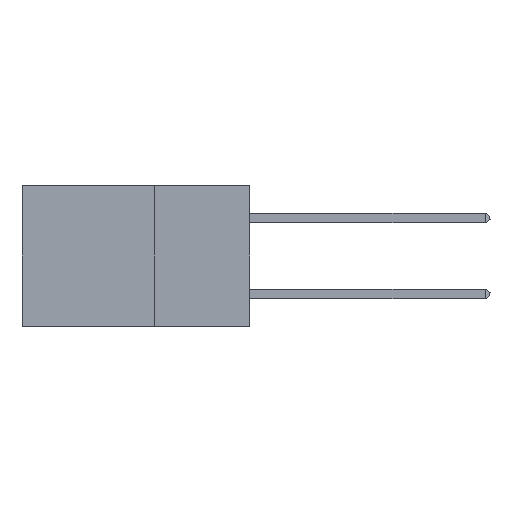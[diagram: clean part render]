
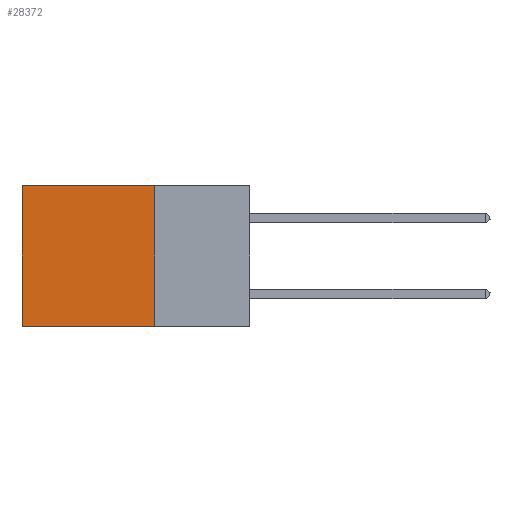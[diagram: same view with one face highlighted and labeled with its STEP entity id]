
A CAD part, left-side view. The second image highlights one B-rep face of the part: STEP entity #28372.
In plain terms, the highlighted planar face has unit normal (-1, 0, 0).
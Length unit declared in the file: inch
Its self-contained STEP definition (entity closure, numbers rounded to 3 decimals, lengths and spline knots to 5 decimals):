
#21 = VECTOR ( 'NONE', #28207, 39.37008 ) ;
#1309 = ORIENTED_EDGE ( 'NONE', *, *, #24073, .F. ) ;
#2085 = CARTESIAN_POINT ( 'NONE',  ( 0.2875, 0.25, -0.37 ) ) ;
#2307 = CARTESIAN_POINT ( 'NONE',  ( 0.2875, 0.6, -0.37 ) ) ;
#4442 = CARTESIAN_POINT ( 'NONE',  ( 0.2875, 0.6, 0. ) ) ;
#6244 = CARTESIAN_POINT ( 'NONE',  ( 0.2875, 0.6, 0. ) ) ;
#6310 = VECTOR ( 'NONE', #12137, 39.37008 ) ;
#8780 = EDGE_CURVE ( 'NONE', #23820, #26030, #32071, .T. ) ;
#9561 = FACE_OUTER_BOUND ( 'NONE', #30292, .T. ) ;
#12137 = DIRECTION ( 'NONE',  ( 0., 0., -1. ) ) ;
#13172 = CARTESIAN_POINT ( 'NONE',  ( 0.2875, 0.25, 0. ) ) ;
#13196 = VECTOR ( 'NONE', #37421, 39.37008 ) ;
#14768 = ORIENTED_EDGE ( 'NONE', *, *, #31474, .T. ) ;
#14882 = VERTEX_POINT ( 'NONE', #2085 ) ;
#15533 = DIRECTION ( 'NONE',  ( 0., 0., -1. ) ) ;
#16046 = ORIENTED_EDGE ( 'NONE', *, *, #35942, .F. ) ;
#16591 = CARTESIAN_POINT ( 'NONE',  ( 0.2875, 0.25, -0.37 ) ) ;
#17099 = ORIENTED_EDGE ( 'NONE', *, *, #8780, .T. ) ;
#18482 = CARTESIAN_POINT ( 'NONE',  ( 0.2875, 0.25, 0. ) ) ;
#20357 = LINE ( 'NONE', #16591, #13196 ) ;
#21575 = PLANE ( 'NONE',  #27815 ) ;
#22110 = LINE ( 'NONE', #6244, #30879 ) ;
#23820 = VERTEX_POINT ( 'NONE', #34903 ) ;
#24073 = EDGE_CURVE ( 'NONE', #23820, #14882, #38143, .T. ) ;
#26030 = VERTEX_POINT ( 'NONE', #4442 ) ;
#26228 = VERTEX_POINT ( 'NONE', #2307 ) ;
#27205 = CARTESIAN_POINT ( 'NONE',  ( 0.2875, 0.25, 0. ) ) ;
#27389 = DIRECTION ( 'NONE',  ( 0., 0., -1. ) ) ;
#27815 = AXIS2_PLACEMENT_3D ( 'NONE', #18482, #33432, #15533 ) ;
#28207 = DIRECTION ( 'NONE',  ( 0., 1., 0. ) ) ;
#28372 = ADVANCED_FACE ( 'NONE', ( #9561 ), #21575, .F. ) ;
#30292 = EDGE_LOOP ( 'NONE', ( #14768, #16046, #1309, #17099 ) ) ;
#30879 = VECTOR ( 'NONE', #27389, 39.37008 ) ;
#31474 = EDGE_CURVE ( 'NONE', #26030, #26228, #22110, .T. ) ;
#32071 = LINE ( 'NONE', #13172, #21 ) ;
#33432 = DIRECTION ( 'NONE',  ( 1., 0., 0. ) ) ;
#34903 = CARTESIAN_POINT ( 'NONE',  ( 0.2875, 0.25, 0. ) ) ;
#35942 = EDGE_CURVE ( 'NONE', #14882, #26228, #20357, .T. ) ;
#37421 = DIRECTION ( 'NONE',  ( 0., 1., 0. ) ) ;
#38143 = LINE ( 'NONE', #27205, #6310 ) ;
